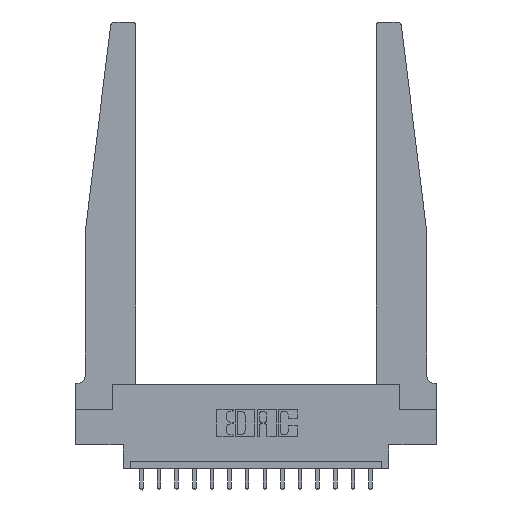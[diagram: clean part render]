
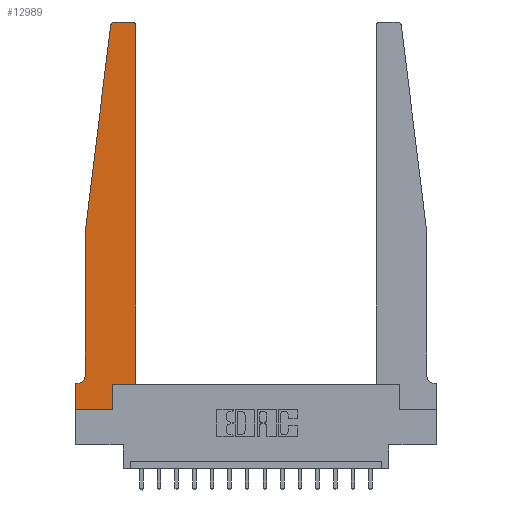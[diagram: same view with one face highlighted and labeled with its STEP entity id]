
A CAD part, top view. The second image highlights one B-rep face of the part: STEP entity #12989.
In plain terms, the highlighted planar face has unit normal (0, 0, 1).
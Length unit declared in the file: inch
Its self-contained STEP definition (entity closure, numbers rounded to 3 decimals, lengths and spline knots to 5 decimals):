
#69 = CARTESIAN_POINT ( 'NONE',  ( 0.425, 0.18, 0.37 ) ) ;
#84 = DIRECTION ( 'NONE',  ( -1., 0., 0. ) ) ;
#265 = VERTEX_POINT ( 'NONE', #2141 ) ;
#330 = VECTOR ( 'NONE', #13535, 39.37008 ) ;
#928 = ORIENTED_EDGE ( 'NONE', *, *, #14541, .T. ) ;
#1077 = LINE ( 'NONE', #16450, #6041 ) ;
#1183 = CARTESIAN_POINT ( 'NONE',  ( 0.27653, 2.75, 0.37 ) ) ;
#1186 = VERTEX_POINT ( 'NONE', #11071 ) ;
#1405 = CARTESIAN_POINT ( 'NONE',  ( 0.25, 2.75, 0.37 ) ) ;
#1741 = DIRECTION ( 'NONE',  ( 1., 0., 0. ) ) ;
#1746 = LINE ( 'NONE', #10603, #7158 ) ;
#1749 = VERTEX_POINT ( 'NONE', #4564 ) ;
#2015 = EDGE_CURVE ( 'NONE', #15098, #1186, #1746, .T. ) ;
#2141 = CARTESIAN_POINT ( 'NONE',  ( 0.24675, 2.72367, 0.37 ) ) ;
#2311 = LINE ( 'NONE', #9585, #11324 ) ;
#2613 = ORIENTED_EDGE ( 'NONE', *, *, #6919, .T. ) ;
#2720 = CARTESIAN_POINT ( 'NONE',  ( 0.065, 1.25, 0.37 ) ) ;
#2723 = AXIS2_PLACEMENT_3D ( 'NONE', #13301, #14797, #9178 ) ;
#3354 = EDGE_CURVE ( 'NONE', #265, #3575, #11240, .T. ) ;
#3493 = CARTESIAN_POINT ( 'NONE',  ( 0.065, 1.25, 0.37 ) ) ;
#3575 = VERTEX_POINT ( 'NONE', #2720 ) ;
#3828 = LINE ( 'NONE', #69, #15847 ) ;
#3937 = DIRECTION ( 'NONE',  ( 1., 0., 0. ) ) ;
#4564 = CARTESIAN_POINT ( 'NONE',  ( 0.2605, 0.18, 0.37 ) ) ;
#4720 = ORIENTED_EDGE ( 'NONE', *, *, #3354, .T. ) ;
#4807 = EDGE_CURVE ( 'NONE', #3575, #5995, #9103, .T. ) ;
#4844 = DIRECTION ( 'NONE',  ( -0.122, -0.992, 0. ) ) ;
#5016 = CARTESIAN_POINT ( 'NONE',  ( 0.065, 1.25, 0.37 ) ) ;
#5199 = CARTESIAN_POINT ( 'NONE',  ( 0., 0.1875, 0.37 ) ) ;
#5399 = AXIS2_PLACEMENT_3D ( 'NONE', #13850, #11230, #1741 ) ;
#5832 = ORIENTED_EDGE ( 'NONE', *, *, #4807, .T. ) ;
#5995 = VERTEX_POINT ( 'NONE', #16251 ) ;
#6041 = VECTOR ( 'NONE', #15146, 39.37008 ) ;
#6062 = CIRCLE ( 'NONE', #2723, 0.05 ) ;
#6428 = EDGE_CURVE ( 'NONE', #1186, #7985, #1077, .T. ) ;
#6453 = ORIENTED_EDGE ( 'NONE', *, *, #9297, .T. ) ;
#6800 = AXIS2_PLACEMENT_3D ( 'NONE', #7924, #17264, #9237 ) ;
#6862 = DIRECTION ( 'NONE',  ( 0., 1., 0. ) ) ;
#6874 = ORIENTED_EDGE ( 'NONE', *, *, #11330, .T. ) ;
#6919 = EDGE_CURVE ( 'NONE', #14628, #15098, #2311, .T. ) ;
#7133 = CARTESIAN_POINT ( 'NONE',  ( 0.425, 2.72, 0.37 ) ) ;
#7158 = VECTOR ( 'NONE', #7885, 39.37008 ) ;
#7186 = VECTOR ( 'NONE', #14144, 39.37008 ) ;
#7508 = FACE_OUTER_BOUND ( 'NONE', #16775, .T. ) ;
#7635 = VERTEX_POINT ( 'NONE', #13325 ) ;
#7885 = DIRECTION ( 'NONE',  ( 0., -1., 0. ) ) ;
#7924 = CARTESIAN_POINT ( 'NONE',  ( 0.395, 2.72, 0.37 ) ) ;
#7955 = EDGE_CURVE ( 'NONE', #12234, #14530, #3828, .T. ) ;
#7985 = VERTEX_POINT ( 'NONE', #16312 ) ;
#9103 = LINE ( 'NONE', #3493, #11783 ) ;
#9131 = CARTESIAN_POINT ( 'NONE',  ( 0.425, 0.18, 0.37 ) ) ;
#9144 = CIRCLE ( 'NONE', #5399, 0.03 ) ;
#9166 = AXIS2_PLACEMENT_3D ( 'NONE', #5199, #11971, #3937 ) ;
#9178 = DIRECTION ( 'NONE',  ( -1., 0., 0. ) ) ;
#9237 = DIRECTION ( 'NONE',  ( 1., 0., 0. ) ) ;
#9250 = EDGE_CURVE ( 'NONE', #14530, #7635, #12321, .T. ) ;
#9297 = EDGE_CURVE ( 'NONE', #7985, #1749, #15294, .T. ) ;
#9585 = CARTESIAN_POINT ( 'NONE',  ( 0.065, 0.1875, 0.37 ) ) ;
#10364 = ORIENTED_EDGE ( 'NONE', *, *, #15110, .T. ) ;
#10603 = CARTESIAN_POINT ( 'NONE',  ( 0., 0., 0.37 ) ) ;
#10793 = LINE ( 'NONE', #15573, #7186 ) ;
#11069 = ORIENTED_EDGE ( 'NONE', *, *, #2015, .T. ) ;
#11071 = CARTESIAN_POINT ( 'NONE',  ( 0., 0., 0.37 ) ) ;
#11118 = ORIENTED_EDGE ( 'NONE', *, *, #9250, .T. ) ;
#11230 = DIRECTION ( 'NONE',  ( 0., 0., 1. ) ) ;
#11240 = LINE ( 'NONE', #5016, #14408 ) ;
#11324 = VECTOR ( 'NONE', #84, 39.37008 ) ;
#11330 = EDGE_CURVE ( 'NONE', #12926, #265, #9144, .T. ) ;
#11427 = CARTESIAN_POINT ( 'NONE',  ( 0.015, 0.1875, 0.37 ) ) ;
#11514 = ORIENTED_EDGE ( 'NONE', *, *, #11889, .T. ) ;
#11783 = VECTOR ( 'NONE', #15622, 39.37008 ) ;
#11889 = EDGE_CURVE ( 'NONE', #7635, #12926, #15454, .T. ) ;
#11971 = DIRECTION ( 'NONE',  ( 0., 0., 1. ) ) ;
#12234 = VERTEX_POINT ( 'NONE', #9131 ) ;
#12321 = CIRCLE ( 'NONE', #6800, 0.03 ) ;
#12926 = VERTEX_POINT ( 'NONE', #1183 ) ;
#12989 = ADVANCED_FACE ( 'NONE', ( #7508 ), #13143, .T. ) ;
#13143 = PLANE ( 'NONE',  #9166 ) ;
#13158 = CARTESIAN_POINT ( 'NONE',  ( 0., 0.1875, 0.37 ) ) ;
#13301 = CARTESIAN_POINT ( 'NONE',  ( 0.015, 0.2375, 0.37 ) ) ;
#13320 = CARTESIAN_POINT ( 'NONE',  ( 0.2605, 0.18, 0.37 ) ) ;
#13325 = CARTESIAN_POINT ( 'NONE',  ( 0.395, 2.75, 0.37 ) ) ;
#13350 = ORIENTED_EDGE ( 'NONE', *, *, #7955, .T. ) ;
#13535 = DIRECTION ( 'NONE',  ( -1., 0., 0. ) ) ;
#13850 = CARTESIAN_POINT ( 'NONE',  ( 0.27653, 2.72, 0.37 ) ) ;
#13878 = DIRECTION ( 'NONE',  ( 0., 1., 0. ) ) ;
#14144 = DIRECTION ( 'NONE',  ( 1., 0., 0. ) ) ;
#14408 = VECTOR ( 'NONE', #4844, 39.37008 ) ;
#14438 = VECTOR ( 'NONE', #13878, 39.37008 ) ;
#14530 = VERTEX_POINT ( 'NONE', #7133 ) ;
#14541 = EDGE_CURVE ( 'NONE', #1749, #12234, #10793, .T. ) ;
#14628 = VERTEX_POINT ( 'NONE', #11427 ) ;
#14797 = DIRECTION ( 'NONE',  ( 0., 0., -1. ) ) ;
#15098 = VERTEX_POINT ( 'NONE', #13158 ) ;
#15110 = EDGE_CURVE ( 'NONE', #5995, #14628, #6062, .T. ) ;
#15146 = DIRECTION ( 'NONE',  ( 1., 0., 0. ) ) ;
#15290 = ORIENTED_EDGE ( 'NONE', *, *, #6428, .T. ) ;
#15294 = LINE ( 'NONE', #13320, #14438 ) ;
#15454 = LINE ( 'NONE', #1405, #330 ) ;
#15573 = CARTESIAN_POINT ( 'NONE',  ( 0.425, 0.18, 0.37 ) ) ;
#15622 = DIRECTION ( 'NONE',  ( 0., -1., 0. ) ) ;
#15847 = VECTOR ( 'NONE', #6862, 39.37008 ) ;
#16251 = CARTESIAN_POINT ( 'NONE',  ( 0.065, 0.2375, 0.37 ) ) ;
#16312 = CARTESIAN_POINT ( 'NONE',  ( 0.2605, 0., 0.37 ) ) ;
#16450 = CARTESIAN_POINT ( 'NONE',  ( 0., 0., 0.37 ) ) ;
#16775 = EDGE_LOOP ( 'NONE', ( #11514, #6874, #4720, #5832, #10364, #2613, #11069, #15290, #6453, #928, #13350, #11118 ) ) ;
#17264 = DIRECTION ( 'NONE',  ( 0., 0., 1. ) ) ;
